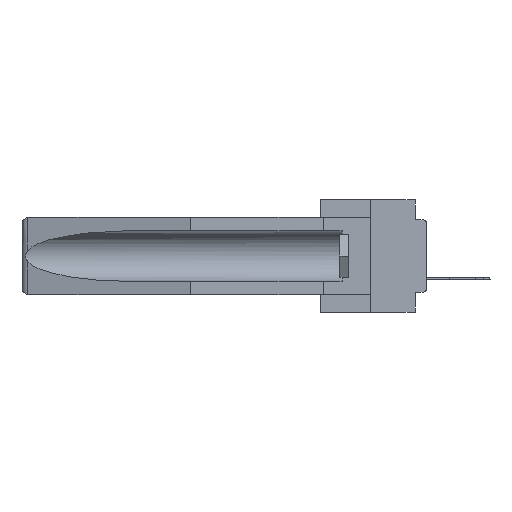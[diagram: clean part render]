
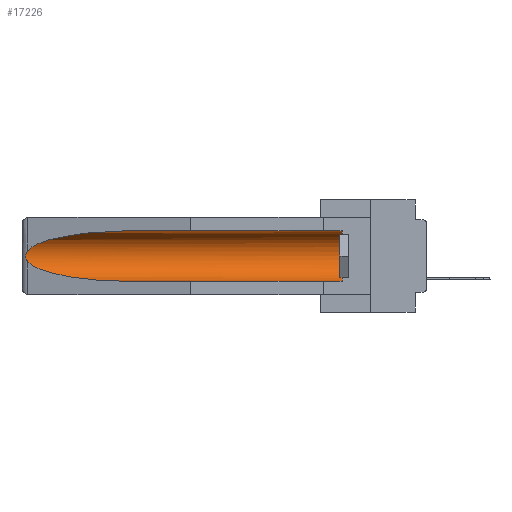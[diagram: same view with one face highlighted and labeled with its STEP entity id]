
A CAD part, left-side view. The second image highlights one B-rep face of the part: STEP entity #17226.
In plain terms, the highlighted cylindrical face has radius 2.857 mm (diameter 5.715 mm), a partial arc.
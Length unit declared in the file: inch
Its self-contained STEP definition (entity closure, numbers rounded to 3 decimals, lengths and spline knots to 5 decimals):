
#178 = EDGE_CURVE ( 'NONE', #21375, #16706, #11039, .T. ) ;
#624 = CARTESIAN_POINT ( 'NONE',  ( 0.21114, 1.30732, -0.059 ) ) ;
#2202 = CARTESIAN_POINT ( 'NONE',  ( 0.155, 1.07973, -0.284 ) ) ;
#2324 = CARTESIAN_POINT ( 'NONE',  ( 0.25451, 1.48313, -0.24835 ) ) ;
#3092 = LINE ( 'NONE', #29366, #20422 ) ;
#3420 = CARTESIAN_POINT ( 'NONE',  ( 0.2675, 1.53308, -0.16763 ) ) ;
#3640 = CARTESIAN_POINT ( 'NONE',  ( 0.2673, 1.5327, -0.16383 ) ) ;
#5318 = CARTESIAN_POINT ( 'NONE',  ( 0.155, 0.126, -0.059 ) ) ;
#5382 = VERTEX_POINT ( 'NONE', #31844 ) ;
#5405 = DIRECTION ( 'NONE',  ( 0., 1., 0. ) ) ;
#5581 = CARTESIAN_POINT ( 'NONE',  ( 0.155, 1.07973, -0.059 ) ) ;
#5887 = EDGE_CURVE ( 'NONE', #13954, #21375, #15908, .T. ) ;
#6046 = CARTESIAN_POINT ( 'NONE',  ( 0.26537, 1.52718, -0.19328 ) ) ;
#7752 = DIRECTION ( 'NONE',  ( 0., -1., 0. ) ) ;
#7865 = EDGE_CURVE ( 'NONE', #17567, #16706, #3092, .T. ) ;
#7891 = CARTESIAN_POINT ( 'NONE',  ( 0.25451, 1.48313, -0.09465 ) ) ;
#8274 = FACE_OUTER_BOUND ( 'NONE', #12490, .T. ) ;
#8720 = CARTESIAN_POINT ( 'NONE',  ( 0.26655, 1.53094, -0.18657 ) ) ;
#9067 = AXIS2_PLACEMENT_3D ( 'NONE', #20318, #7752, #20435 ) ;
#9940 = ORIENTED_EDGE ( 'NONE', *, *, #7865, .F. ) ;
#11039 =( BOUNDED_CURVE ( )  B_SPLINE_CURVE ( 3, ( #22391, #2324, #22494, #2202 ),
 .UNSPECIFIED., .F., .F. ) 
 B_SPLINE_CURVE_WITH_KNOTS ( ( 4, 4 ),
 ( 0.1948, 1.5708 ),
 .UNSPECIFIED. ) 
 CURVE ( )  GEOMETRIC_REPRESENTATION_ITEM ( )  RATIONAL_B_SPLINE_CURVE ( ( 1., 0.848, 0.848, 1. ) ) 
 REPRESENTATION_ITEM ( '' )  );
#11041 = CARTESIAN_POINT ( 'NONE',  ( 0.26654, 1.53092, -0.15636 ) ) ;
#12135 = DIRECTION ( 'NONE',  ( 0., 1., 0. ) ) ;
#12490 = EDGE_LOOP ( 'NONE', ( #15065, #30124, #14302, #9940, #15750, #17916 ) ) ;
#13602 = CARTESIAN_POINT ( 'NONE',  ( 0.155, 1.07973, -0.284 ) ) ;
#13931 = CARTESIAN_POINT ( 'NONE',  ( 0.26597, 1.52961, -0.15275 ) ) ;
#13954 = VERTEX_POINT ( 'NONE', #23481 ) ;
#14302 = ORIENTED_EDGE ( 'NONE', *, *, #178, .T. ) ;
#14624 =( BOUNDED_CURVE ( )  B_SPLINE_CURVE ( 3, ( #5581, #624, #7891, #24471 ),
 .UNSPECIFIED., .F., .F. ) 
 B_SPLINE_CURVE_WITH_KNOTS ( ( 4, 4 ),
 ( 4.71239, 6.08839 ),
 .UNSPECIFIED. ) 
 CURVE ( )  GEOMETRIC_REPRESENTATION_ITEM ( )  RATIONAL_B_SPLINE_CURVE ( ( 1., 0.848, 0.848, 1. ) ) 
 REPRESENTATION_ITEM ( '' )  );
#14644 = LINE ( 'NONE', #17821, #15461 ) ;
#15065 = ORIENTED_EDGE ( 'NONE', *, *, #18064, .T. ) ;
#15461 = VECTOR ( 'NONE', #22509, 39.37008 ) ;
#15750 = ORIENTED_EDGE ( 'NONE', *, *, #16743, .T. ) ;
#15908 = B_SPLINE_CURVE_WITH_KNOTS ( 'NONE', 3,
 ( #16361, #13931, #11041, #3640, #3420, #28593, #21279, #8720, #31434, #6046 ),
 .UNSPECIFIED., .F., .F.,
 ( 4, 2, 2, 2, 4 ),
 ( 0., 0.00029, 0.00058, 0.00087, 0.00117 ),
 .UNSPECIFIED. ) ;
#16361 = CARTESIAN_POINT ( 'NONE',  ( 0.26537, 1.52718, -0.14972 ) ) ;
#16706 = VERTEX_POINT ( 'NONE', #13602 ) ;
#16743 = EDGE_CURVE ( 'NONE', #17567, #25755, #25292, .T. ) ;
#17226 = ADVANCED_FACE ( 'NONE', ( #8274 ), #31062, .F. ) ;
#17567 = VERTEX_POINT ( 'NONE', #28578 ) ;
#17821 = CARTESIAN_POINT ( 'NONE',  ( 0.155, -0.30754, -0.059 ) ) ;
#17916 = ORIENTED_EDGE ( 'NONE', *, *, #23857, .T. ) ;
#18064 = EDGE_CURVE ( 'NONE', #5382, #13954, #14624, .T. ) ;
#20318 = CARTESIAN_POINT ( 'NONE',  ( 0.155, 0.126, -0.1715 ) ) ;
#20422 = VECTOR ( 'NONE', #12135, 39.37008 ) ;
#20435 = DIRECTION ( 'NONE',  ( 0., 0., 1. ) ) ;
#21279 = CARTESIAN_POINT ( 'NONE',  ( 0.2673, 1.53269, -0.17917 ) ) ;
#21375 = VERTEX_POINT ( 'NONE', #31863 ) ;
#22391 = CARTESIAN_POINT ( 'NONE',  ( 0.26537, 1.52718, -0.19328 ) ) ;
#22494 = CARTESIAN_POINT ( 'NONE',  ( 0.21114, 1.30732, -0.284 ) ) ;
#22509 = DIRECTION ( 'NONE',  ( 0., 1., 0. ) ) ;
#22932 = CARTESIAN_POINT ( 'NONE',  ( 0.155, -0.30754, -0.1715 ) ) ;
#23481 = CARTESIAN_POINT ( 'NONE',  ( 0.26537, 1.52718, -0.14972 ) ) ;
#23857 = EDGE_CURVE ( 'NONE', #25755, #5382, #14644, .T. ) ;
#24471 = CARTESIAN_POINT ( 'NONE',  ( 0.26537, 1.52718, -0.14972 ) ) ;
#24863 = AXIS2_PLACEMENT_3D ( 'NONE', #22932, #5405, #25573 ) ;
#25292 = CIRCLE ( 'NONE', #9067, 0.1125 ) ;
#25573 = DIRECTION ( 'NONE',  ( 0., 0., 1. ) ) ;
#25755 = VERTEX_POINT ( 'NONE', #5318 ) ;
#28578 = CARTESIAN_POINT ( 'NONE',  ( 0.155, 0.126, -0.284 ) ) ;
#28593 = CARTESIAN_POINT ( 'NONE',  ( 0.2675, 1.53308, -0.17534 ) ) ;
#29366 = CARTESIAN_POINT ( 'NONE',  ( 0.155, -0.30754, -0.284 ) ) ;
#30124 = ORIENTED_EDGE ( 'NONE', *, *, #5887, .T. ) ;
#31062 = CYLINDRICAL_SURFACE ( 'NONE', #24863, 0.1125 ) ;
#31434 = CARTESIAN_POINT ( 'NONE',  ( 0.26597, 1.5296, -0.19026 ) ) ;
#31844 = CARTESIAN_POINT ( 'NONE',  ( 0.155, 1.07973, -0.059 ) ) ;
#31863 = CARTESIAN_POINT ( 'NONE',  ( 0.26537, 1.52718, -0.19328 ) ) ;
